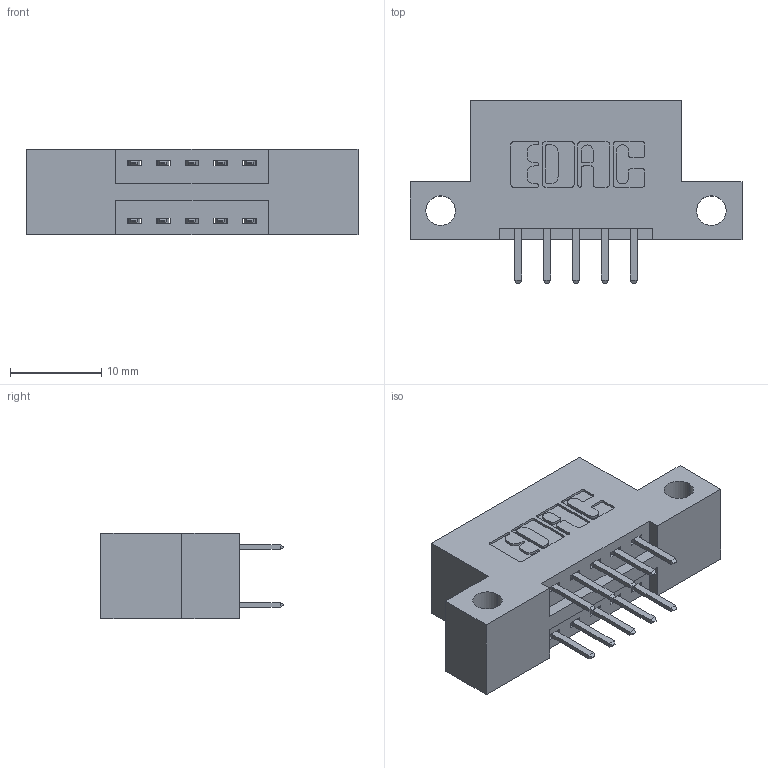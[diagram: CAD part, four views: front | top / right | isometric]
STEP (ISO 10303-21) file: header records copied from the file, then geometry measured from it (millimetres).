
FILE_DESCRIPTION (( 'STEP AP203' ), '1' );
FILE_NAME ('346-010-520-212.STEP', '2018-08-17T06:25:10', ( '' ), ( '' ), 'SwSTEP 2.0', 'SolidWorks 2016', '' );
FILE_SCHEMA (( 'CONFIG_CONTROL_DESIGN' ));
Length unit declared in the file: inch
Products named in the file (3): 346 Part_Flush Mounting Lugs - Side Mount; 345-292-001_345-293-120; 346-010-520-212
Assembly tree (11 placements, depth 2):
  346-010-520-212
    346 Part_Flush Mounting Lugs - Side Mount
    345-292-001_345-293-120  x10
Bounding box: 36.45 x 20.02 x 9.4 mm (x, y, z)
Volume: 3175.2 mm3; surface area: 3635.2 mm2
Topology: 11 solids, 11 shells, 682 faces, 1959 edges, 1278 vertices
Faces by surface type: plane 446, cylinder 236
Entity records: 8361 total; most frequent: CARTESIAN_POINT 1440, ORIENTED_EDGE 1362, DIRECTION 1309, EDGE_CURVE 681, LINE 525, VECTOR 525, VERTEX_POINT 450, AXIS2_PLACEMENT_3D 392
